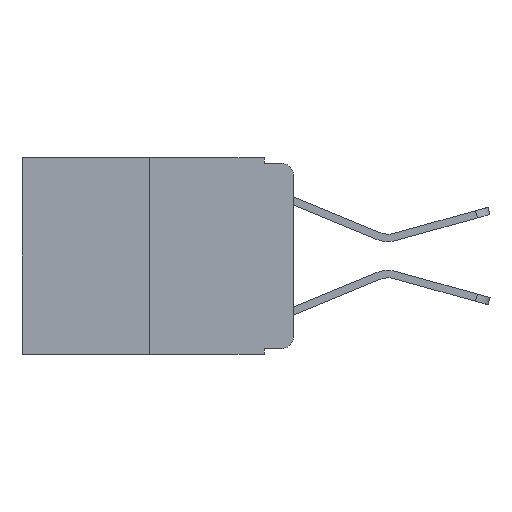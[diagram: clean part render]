
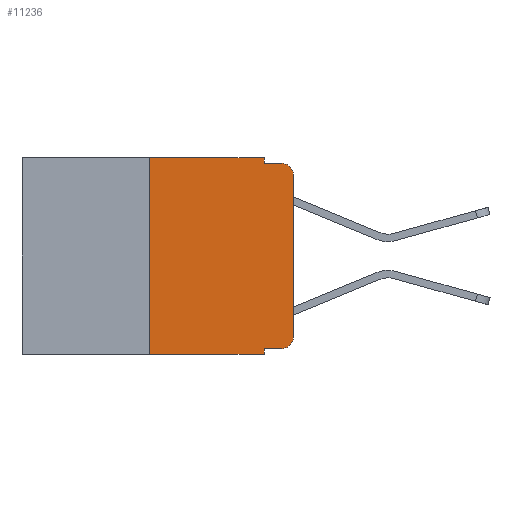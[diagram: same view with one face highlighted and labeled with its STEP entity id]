
A CAD part, left-side view. The second image highlights one B-rep face of the part: STEP entity #11236.
In plain terms, the highlighted planar face has unit normal (-1, 0, 0).
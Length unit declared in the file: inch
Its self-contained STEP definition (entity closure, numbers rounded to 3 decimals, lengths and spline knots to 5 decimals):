
#216 = DIRECTION ( 'NONE',  ( 0., 0., 1. ) ) ;
#531 = VERTEX_POINT ( 'NONE', #13536 ) ;
#694 = VERTEX_POINT ( 'NONE', #2760 ) ;
#991 = EDGE_CURVE ( 'NONE', #5386, #14012, #14514, .T. ) ;
#1062 = AXIS2_PLACEMENT_3D ( 'NONE', #3543, #8331, #15668 ) ;
#1111 = EDGE_LOOP ( 'NONE', ( #10152, #2208, #3312, #12080, #12498, #2003, #15147, #15474, #14071, #6035 ) ) ;
#1125 = DIRECTION ( 'NONE',  ( -1., 0., 0. ) ) ;
#1217 = DIRECTION ( 'NONE',  ( 0., -1., 0. ) ) ;
#1366 = VECTOR ( 'NONE', #9019, 39.37008 ) ;
#1584 = CIRCLE ( 'NONE', #3600, 0.02 ) ;
#1640 = FACE_OUTER_BOUND ( 'NONE', #1111, .T. ) ;
#1863 = CARTESIAN_POINT ( 'NONE',  ( 0., 0.051, 0. ) ) ;
#2003 = ORIENTED_EDGE ( 'NONE', *, *, #14929, .F. ) ;
#2061 = DIRECTION ( 'NONE',  ( 0., 0., -1. ) ) ;
#2197 = CARTESIAN_POINT ( 'NONE',  ( 0., 0.051, -0.01 ) ) ;
#2208 = ORIENTED_EDGE ( 'NONE', *, *, #13529, .T. ) ;
#2760 = CARTESIAN_POINT ( 'NONE',  ( 0., 0.02, -0.01 ) ) ;
#2879 = EDGE_CURVE ( 'NONE', #10889, #15084, #10664, .T. ) ;
#3312 = ORIENTED_EDGE ( 'NONE', *, *, #12569, .F. ) ;
#3477 = VECTOR ( 'NONE', #9814, 39.37008 ) ;
#3543 = CARTESIAN_POINT ( 'NONE',  ( 0., 0.473, 0. ) ) ;
#3600 = AXIS2_PLACEMENT_3D ( 'NONE', #14110, #15310, #2061 ) ;
#3672 = CARTESIAN_POINT ( 'NONE',  ( 0., 0.473, -0.343 ) ) ;
#3816 = LINE ( 'NONE', #3672, #14274 ) ;
#3851 = CARTESIAN_POINT ( 'NONE',  ( 0., 0.051, -0.333 ) ) ;
#4247 = LINE ( 'NONE', #4763, #3477 ) ;
#4419 = VERTEX_POINT ( 'NONE', #10934 ) ;
#4763 = CARTESIAN_POINT ( 'NONE',  ( 0., 0.051, -0.01 ) ) ;
#4813 = CARTESIAN_POINT ( 'NONE',  ( 0., 0., 0. ) ) ;
#5036 = DIRECTION ( 'NONE',  ( 0., -1., 0. ) ) ;
#5162 = VECTOR ( 'NONE', #6944, 39.37008 ) ;
#5175 = LINE ( 'NONE', #3851, #7242 ) ;
#5386 = VERTEX_POINT ( 'NONE', #6836 ) ;
#6035 = ORIENTED_EDGE ( 'NONE', *, *, #13028, .T. ) ;
#6268 = EDGE_CURVE ( 'NONE', #10726, #15084, #3816, .T. ) ;
#6836 = CARTESIAN_POINT ( 'NONE',  ( 0., 0.25, 0. ) ) ;
#6925 = EDGE_CURVE ( 'NONE', #4419, #531, #14801, .T. ) ;
#6944 = DIRECTION ( 'NONE',  ( 0., 0., -1. ) ) ;
#7242 = VECTOR ( 'NONE', #1217, 39.37008 ) ;
#7484 = CARTESIAN_POINT ( 'NONE',  ( 0., 0.25, 0. ) ) ;
#7582 = VECTOR ( 'NONE', #216, 39.37008 ) ;
#8074 = CARTESIAN_POINT ( 'NONE',  ( 0., 0.051, 0. ) ) ;
#8331 = DIRECTION ( 'NONE',  ( 1., 0., 0. ) ) ;
#8371 = VECTOR ( 'NONE', #13423, 39.37008 ) ;
#8385 = PLANE ( 'NONE',  #1062 ) ;
#8389 = CARTESIAN_POINT ( 'NONE',  ( 0., 0.02, -0.313 ) ) ;
#8799 = CARTESIAN_POINT ( 'NONE',  ( 0., 0.02, -0.333 ) ) ;
#9019 = DIRECTION ( 'NONE',  ( 0., 0., -1. ) ) ;
#9150 = LINE ( 'NONE', #1863, #1366 ) ;
#9814 = DIRECTION ( 'NONE',  ( 0., -1., 0. ) ) ;
#10152 = ORIENTED_EDGE ( 'NONE', *, *, #6925, .T. ) ;
#10516 = CIRCLE ( 'NONE', #12267, 0.02 ) ;
#10664 = LINE ( 'NONE', #8074, #5162 ) ;
#10726 = VERTEX_POINT ( 'NONE', #14959 ) ;
#10818 = DIRECTION ( 'NONE',  ( 0., 0., -1. ) ) ;
#10889 = VERTEX_POINT ( 'NONE', #13543 ) ;
#10934 = CARTESIAN_POINT ( 'NONE',  ( 0., 0., -0.313 ) ) ;
#11236 = ADVANCED_FACE ( 'NONE', ( #1640 ), #8385, .F. ) ;
#11285 = VECTOR ( 'NONE', #5036, 39.37008 ) ;
#11561 = CARTESIAN_POINT ( 'NONE',  ( 0., 0.051, 0. ) ) ;
#12080 = ORIENTED_EDGE ( 'NONE', *, *, #13916, .F. ) ;
#12267 = AXIS2_PLACEMENT_3D ( 'NONE', #8389, #1125, #10818 ) ;
#12269 = CARTESIAN_POINT ( 'NONE',  ( 0., 0.473, 0. ) ) ;
#12498 = ORIENTED_EDGE ( 'NONE', *, *, #991, .F. ) ;
#12514 = VERTEX_POINT ( 'NONE', #2197 ) ;
#12569 = EDGE_CURVE ( 'NONE', #12514, #694, #4247, .T. ) ;
#13028 = EDGE_CURVE ( 'NONE', #13775, #4419, #10516, .T. ) ;
#13389 = DIRECTION ( 'NONE',  ( 0., -1., 0. ) ) ;
#13423 = DIRECTION ( 'NONE',  ( 0., 0., 1. ) ) ;
#13529 = EDGE_CURVE ( 'NONE', #531, #694, #1584, .T. ) ;
#13536 = CARTESIAN_POINT ( 'NONE',  ( 0., 0., -0.03 ) ) ;
#13543 = CARTESIAN_POINT ( 'NONE',  ( 0., 0.051, -0.333 ) ) ;
#13775 = VERTEX_POINT ( 'NONE', #8799 ) ;
#13786 = EDGE_CURVE ( 'NONE', #10889, #13775, #5175, .T. ) ;
#13916 = EDGE_CURVE ( 'NONE', #14012, #12514, #9150, .T. ) ;
#14012 = VERTEX_POINT ( 'NONE', #11561 ) ;
#14071 = ORIENTED_EDGE ( 'NONE', *, *, #13786, .T. ) ;
#14110 = CARTESIAN_POINT ( 'NONE',  ( 0., 0.02, -0.03 ) ) ;
#14274 = VECTOR ( 'NONE', #13389, 39.37008 ) ;
#14514 = LINE ( 'NONE', #12269, #11285 ) ;
#14801 = LINE ( 'NONE', #4813, #8371 ) ;
#14929 = EDGE_CURVE ( 'NONE', #10726, #5386, #15355, .T. ) ;
#14959 = CARTESIAN_POINT ( 'NONE',  ( 0., 0.25, -0.343 ) ) ;
#15007 = CARTESIAN_POINT ( 'NONE',  ( 0., 0.051, -0.343 ) ) ;
#15084 = VERTEX_POINT ( 'NONE', #15007 ) ;
#15147 = ORIENTED_EDGE ( 'NONE', *, *, #6268, .T. ) ;
#15310 = DIRECTION ( 'NONE',  ( -1., 0., 0. ) ) ;
#15355 = LINE ( 'NONE', #7484, #7582 ) ;
#15474 = ORIENTED_EDGE ( 'NONE', *, *, #2879, .F. ) ;
#15668 = DIRECTION ( 'NONE',  ( 0., 0., -1. ) ) ;
